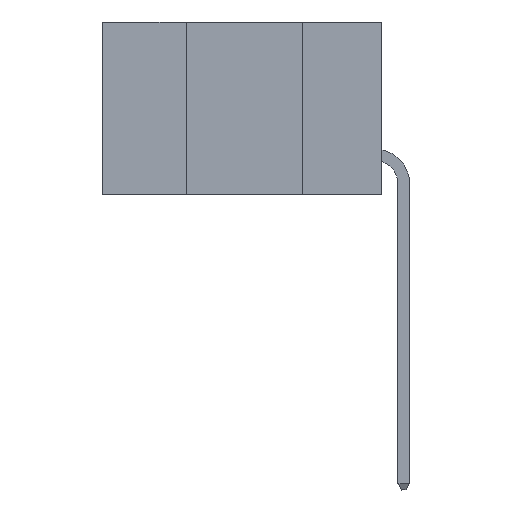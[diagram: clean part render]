
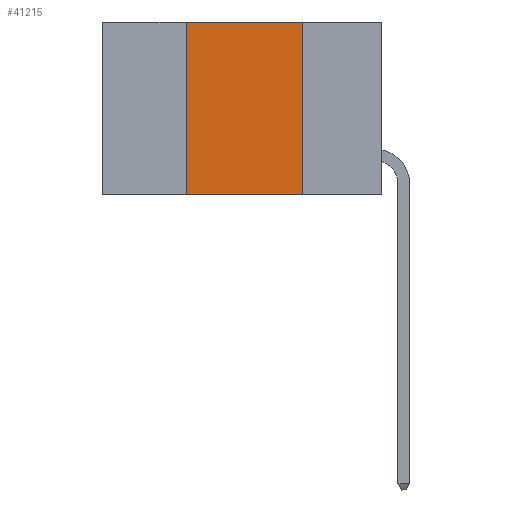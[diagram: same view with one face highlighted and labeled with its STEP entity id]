
A CAD part, left-side view. The second image highlights one B-rep face of the part: STEP entity #41215.
In plain terms, the highlighted planar face has unit normal (-1, 0, 0).
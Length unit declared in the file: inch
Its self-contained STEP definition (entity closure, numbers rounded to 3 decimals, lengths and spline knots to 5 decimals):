
#277 = CARTESIAN_POINT ( 'NONE',  ( 0., 0.17, 0. ) ) ;
#3079 = FACE_OUTER_BOUND ( 'NONE', #3926, .T. ) ;
#3224 = AXIS2_PLACEMENT_3D ( 'NONE', #47994, #36682, #13673 ) ;
#3926 = EDGE_LOOP ( 'NONE', ( #20980, #26429, #38484, #12626 ) ) ;
#4189 = VERTEX_POINT ( 'NONE', #277 ) ;
#7578 = VECTOR ( 'NONE', #9901, 39.37008 ) ;
#7587 = DIRECTION ( 'NONE',  ( 0., 0., 1. ) ) ;
#9745 = PLANE ( 'NONE',  #3224 ) ;
#9901 = DIRECTION ( 'NONE',  ( 0., -1., 0. ) ) ;
#11690 = CARTESIAN_POINT ( 'NONE',  ( 0., 0.42, -0.37 ) ) ;
#12626 = ORIENTED_EDGE ( 'NONE', *, *, #24440, .T. ) ;
#12763 = VECTOR ( 'NONE', #39388, 39.37008 ) ;
#13673 = DIRECTION ( 'NONE',  ( 0., 0., -1. ) ) ;
#13879 = VERTEX_POINT ( 'NONE', #11690 ) ;
#15477 = CARTESIAN_POINT ( 'NONE',  ( 0., 0.42, 0. ) ) ;
#16443 = LINE ( 'NONE', #26560, #36893 ) ;
#17378 = CARTESIAN_POINT ( 'NONE',  ( 0., 0.17, -0.37 ) ) ;
#20980 = ORIENTED_EDGE ( 'NONE', *, *, #48854, .F. ) ;
#23116 = CARTESIAN_POINT ( 'NONE',  ( 0., 0.42, 0. ) ) ;
#24440 = EDGE_CURVE ( 'NONE', #13879, #48636, #26867, .T. ) ;
#26429 = ORIENTED_EDGE ( 'NONE', *, *, #29953, .F. ) ;
#26560 = CARTESIAN_POINT ( 'NONE',  ( 0., 0.17, 0. ) ) ;
#26867 = LINE ( 'NONE', #36818, #7578 ) ;
#29953 = EDGE_CURVE ( 'NONE', #30447, #4189, #43411, .T. ) ;
#30447 = VERTEX_POINT ( 'NONE', #15477 ) ;
#36334 = EDGE_CURVE ( 'NONE', #13879, #30447, #49272, .T. ) ;
#36682 = DIRECTION ( 'NONE',  ( 1., 0., 0. ) ) ;
#36818 = CARTESIAN_POINT ( 'NONE',  ( 0., 0.6, -0.37 ) ) ;
#36893 = VECTOR ( 'NONE', #45659, 39.37008 ) ;
#38484 = ORIENTED_EDGE ( 'NONE', *, *, #36334, .F. ) ;
#39388 = DIRECTION ( 'NONE',  ( 0., -1., 0. ) ) ;
#41215 = ADVANCED_FACE ( 'NONE', ( #3079 ), #9745, .F. ) ;
#43205 = CARTESIAN_POINT ( 'NONE',  ( 0., 0.6, 0. ) ) ;
#43411 = LINE ( 'NONE', #43205, #12763 ) ;
#45659 = DIRECTION ( 'NONE',  ( 0., 0., -1. ) ) ;
#47994 = CARTESIAN_POINT ( 'NONE',  ( 0., 0.6, 0. ) ) ;
#48109 = VECTOR ( 'NONE', #7587, 39.37008 ) ;
#48636 = VERTEX_POINT ( 'NONE', #17378 ) ;
#48854 = EDGE_CURVE ( 'NONE', #4189, #48636, #16443, .T. ) ;
#49272 = LINE ( 'NONE', #23116, #48109 ) ;
